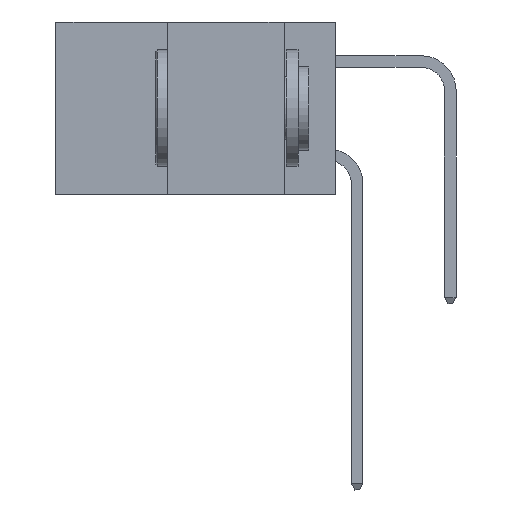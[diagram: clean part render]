
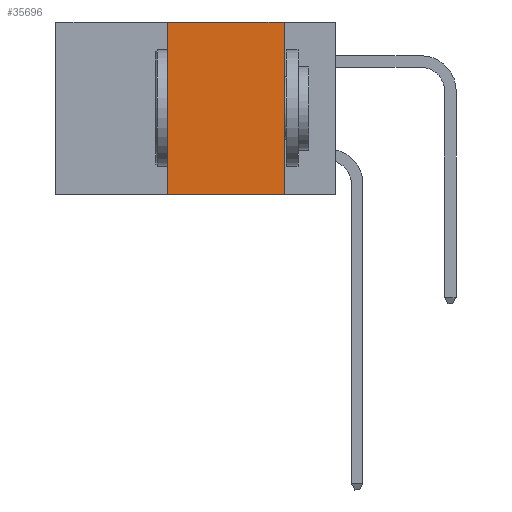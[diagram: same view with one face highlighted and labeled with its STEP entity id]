
A CAD part, left-side view. The second image highlights one B-rep face of the part: STEP entity #35696.
In plain terms, the highlighted planar face has unit normal (-1, 0, 0).
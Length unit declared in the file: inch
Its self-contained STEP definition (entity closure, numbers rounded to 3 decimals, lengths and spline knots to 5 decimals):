
#202 = DIRECTION ( 'NONE',  ( 0., 0., -1. ) ) ;
#1025 = EDGE_CURVE ( 'NONE', #25110, #39678, #11111, .T. ) ;
#1316 = EDGE_CURVE ( 'NONE', #2840, #39678, #4008, .T. ) ;
#1931 = EDGE_CURVE ( 'NONE', #27073, #25110, #24141, .T. ) ;
#2225 = ORIENTED_EDGE ( 'NONE', *, *, #1025, .F. ) ;
#2840 = VERTEX_POINT ( 'NONE', #37523 ) ;
#2899 = LINE ( 'NONE', #34366, #17581 ) ;
#4008 = LINE ( 'NONE', #41186, #19826 ) ;
#4320 = CARTESIAN_POINT ( 'NONE',  ( 0., 0.11, 0. ) ) ;
#7878 = DIRECTION ( 'NONE',  ( 0., 0., -1. ) ) ;
#7959 = FACE_OUTER_BOUND ( 'NONE', #42840, .T. ) ;
#8467 = DIRECTION ( 'NONE',  ( 0., -1., 0. ) ) ;
#11111 = LINE ( 'NONE', #4320, #18755 ) ;
#11519 = DIRECTION ( 'NONE',  ( 1., 0., 0. ) ) ;
#13309 = DIRECTION ( 'NONE',  ( 0., 0., 1. ) ) ;
#13436 = CARTESIAN_POINT ( 'NONE',  ( 0., 0.11, 0. ) ) ;
#17581 = VECTOR ( 'NONE', #13309, 39.37008 ) ;
#18755 = VECTOR ( 'NONE', #202, 39.37008 ) ;
#19826 = VECTOR ( 'NONE', #44830, 39.37008 ) ;
#20311 = VECTOR ( 'NONE', #8467, 39.37008 ) ;
#22755 = EDGE_CURVE ( 'NONE', #2840, #27073, #2899, .T. ) ;
#24141 = LINE ( 'NONE', #42795, #20311 ) ;
#25110 = VERTEX_POINT ( 'NONE', #13436 ) ;
#27073 = VERTEX_POINT ( 'NONE', #39013 ) ;
#31888 = PLANE ( 'NONE',  #43484 ) ;
#34032 = ORIENTED_EDGE ( 'NONE', *, *, #1316, .T. ) ;
#34366 = CARTESIAN_POINT ( 'NONE',  ( 0., 0.36, 0. ) ) ;
#34868 = CARTESIAN_POINT ( 'NONE',  ( 0., 0.11, -0.37 ) ) ;
#35696 = ADVANCED_FACE ( 'NONE', ( #7959 ), #31888, .F. ) ;
#36182 = ORIENTED_EDGE ( 'NONE', *, *, #22755, .F. ) ;
#37523 = CARTESIAN_POINT ( 'NONE',  ( 0., 0.36, -0.37 ) ) ;
#39013 = CARTESIAN_POINT ( 'NONE',  ( 0., 0.36, 0. ) ) ;
#39178 = CARTESIAN_POINT ( 'NONE',  ( 0., 0.6, 0. ) ) ;
#39678 = VERTEX_POINT ( 'NONE', #34868 ) ;
#40542 = ORIENTED_EDGE ( 'NONE', *, *, #1931, .F. ) ;
#41186 = CARTESIAN_POINT ( 'NONE',  ( 0., 0.6, -0.37 ) ) ;
#42795 = CARTESIAN_POINT ( 'NONE',  ( 0., 0.6, 0. ) ) ;
#42840 = EDGE_LOOP ( 'NONE', ( #2225, #40542, #36182, #34032 ) ) ;
#43484 = AXIS2_PLACEMENT_3D ( 'NONE', #39178, #11519, #7878 ) ;
#44830 = DIRECTION ( 'NONE',  ( 0., -1., 0. ) ) ;
